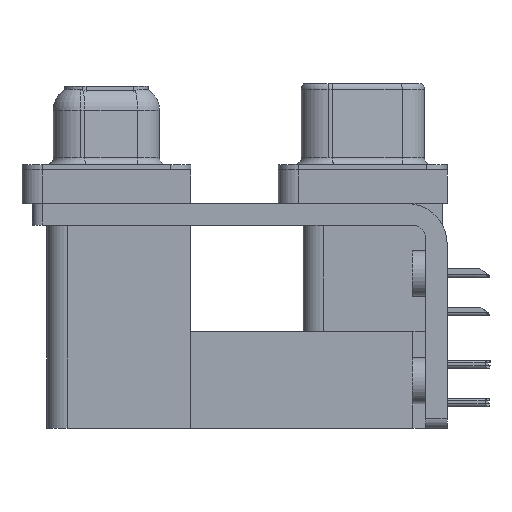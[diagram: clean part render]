
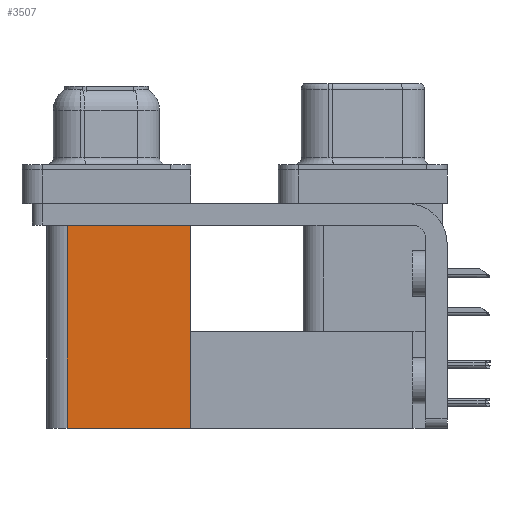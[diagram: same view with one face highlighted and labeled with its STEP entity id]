
A CAD part, left-side view. The second image highlights one B-rep face of the part: STEP entity #3507.
In plain terms, the highlighted planar face has unit normal (-1, 0, 0).
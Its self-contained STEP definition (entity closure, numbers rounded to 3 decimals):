
#250 = VECTOR ( 'NONE', #24742, 1000. ) ;
#3507 = ADVANCED_FACE ( 'NONE', ( #42925 ), #4159, .F. ) ;
#3596 = CARTESIAN_POINT ( 'NONE',  ( 3.765, 21.975, -2.5 ) ) ;
#4159 = PLANE ( 'NONE',  #11783 ) ;
#5745 = EDGE_LOOP ( 'NONE', ( #22670, #29804, #34184, #45982 ) ) ;
#7125 = LINE ( 'NONE', #10428, #250 ) ;
#7239 = VECTOR ( 'NONE', #16753, 1000. ) ;
#7686 = DIRECTION ( 'NONE',  ( 1., 0., 0. ) ) ;
#9259 = LINE ( 'NONE', #10191, #7239 ) ;
#10191 = CARTESIAN_POINT ( 'NONE',  ( 3.765, 12.775, -2.5 ) ) ;
#10428 = CARTESIAN_POINT ( 'NONE',  ( 3.765, 21.975, -19.2 ) ) ;
#11783 = AXIS2_PLACEMENT_3D ( 'NONE', #36567, #7686, #35859 ) ;
#14778 = VERTEX_POINT ( 'NONE', #33301 ) ;
#16753 = DIRECTION ( 'NONE',  ( 0., 1., 0. ) ) ;
#20196 = EDGE_CURVE ( 'NONE', #14778, #43868, #9259, .T. ) ;
#22581 = VECTOR ( 'NONE', #23512, 1000. ) ;
#22670 = ORIENTED_EDGE ( 'NONE', *, *, #20196, .T. ) ;
#23333 = DIRECTION ( 'NONE',  ( 0., 1., 0. ) ) ;
#23512 = DIRECTION ( 'NONE',  ( 0., 0., 1. ) ) ;
#24742 = DIRECTION ( 'NONE',  ( 0., 0., 1. ) ) ;
#25638 = EDGE_CURVE ( 'NONE', #26721, #14778, #45824, .T. ) ;
#26721 = VERTEX_POINT ( 'NONE', #32217 ) ;
#26874 = CARTESIAN_POINT ( 'NONE',  ( 3.765, 12.775, -19.2 ) ) ;
#28823 = VECTOR ( 'NONE', #23333, 1000. ) ;
#29804 = ORIENTED_EDGE ( 'NONE', *, *, #45956, .F. ) ;
#32217 = CARTESIAN_POINT ( 'NONE',  ( 3.765, 12.775, -19.2 ) ) ;
#33301 = CARTESIAN_POINT ( 'NONE',  ( 3.765, 12.775, -2.5 ) ) ;
#34184 = ORIENTED_EDGE ( 'NONE', *, *, #42795, .F. ) ;
#35426 = VERTEX_POINT ( 'NONE', #40291 ) ;
#35859 = DIRECTION ( 'NONE',  ( 0., 1., 0. ) ) ;
#36567 = CARTESIAN_POINT ( 'NONE',  ( 3.765, 12.775, -19.2 ) ) ;
#37827 = CARTESIAN_POINT ( 'NONE',  ( 3.765, 12.775, -19.2 ) ) ;
#40291 = CARTESIAN_POINT ( 'NONE',  ( 3.765, 21.975, -19.2 ) ) ;
#40497 = LINE ( 'NONE', #26874, #28823 ) ;
#42795 = EDGE_CURVE ( 'NONE', #26721, #35426, #40497, .T. ) ;
#42925 = FACE_OUTER_BOUND ( 'NONE', #5745, .T. ) ;
#43868 = VERTEX_POINT ( 'NONE', #3596 ) ;
#45824 = LINE ( 'NONE', #37827, #22581 ) ;
#45956 = EDGE_CURVE ( 'NONE', #35426, #43868, #7125, .T. ) ;
#45982 = ORIENTED_EDGE ( 'NONE', *, *, #25638, .T. ) ;
